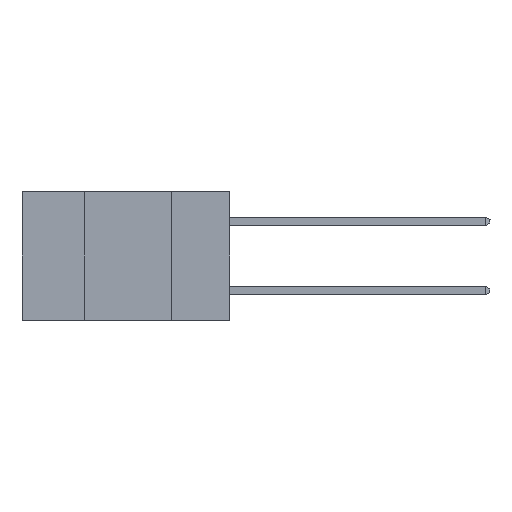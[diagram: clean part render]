
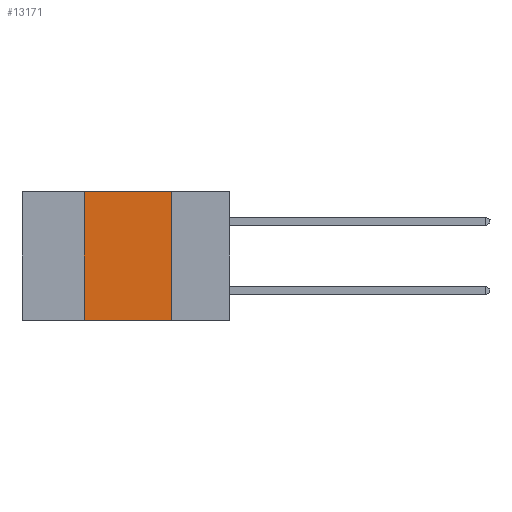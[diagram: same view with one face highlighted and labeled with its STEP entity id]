
A CAD part, left-side view. The second image highlights one B-rep face of the part: STEP entity #13171.
In plain terms, the highlighted planar face has unit normal (-1, 0, 0).
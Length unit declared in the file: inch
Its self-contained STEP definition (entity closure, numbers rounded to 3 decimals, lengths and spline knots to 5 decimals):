
#165 = CARTESIAN_POINT ( 'NONE',  ( 0., 0.42, -0.37 ) ) ;
#690 = VERTEX_POINT ( 'NONE', #16323 ) ;
#1790 = VECTOR ( 'NONE', #17800, 39.37008 ) ;
#2036 = CARTESIAN_POINT ( 'NONE',  ( 0., 0.17, -0.37 ) ) ;
#2674 = VECTOR ( 'NONE', #5970, 39.37008 ) ;
#3017 = EDGE_LOOP ( 'NONE', ( #17303, #17016, #16167, #13512 ) ) ;
#3249 = LINE ( 'NONE', #2036, #5496 ) ;
#3418 = CARTESIAN_POINT ( 'NONE',  ( 0., 0.42, 0. ) ) ;
#3550 = LINE ( 'NONE', #8054, #8302 ) ;
#4145 = EDGE_CURVE ( 'NONE', #10075, #17741, #3249, .T. ) ;
#4650 = CARTESIAN_POINT ( 'NONE',  ( 0., 0.17, -0.37 ) ) ;
#5496 = VECTOR ( 'NONE', #7744, 39.37008 ) ;
#5970 = DIRECTION ( 'NONE',  ( 0., 0., 1. ) ) ;
#6287 = CARTESIAN_POINT ( 'NONE',  ( 0., 0.17, 0. ) ) ;
#7280 = EDGE_CURVE ( 'NONE', #690, #11026, #10277, .T. ) ;
#7514 = FACE_OUTER_BOUND ( 'NONE', #3017, .T. ) ;
#7744 = DIRECTION ( 'NONE',  ( 0., 0., -1. ) ) ;
#7784 = EDGE_CURVE ( 'NONE', #11026, #10075, #7986, .T. ) ;
#7986 = LINE ( 'NONE', #16309, #1790 ) ;
#8054 = CARTESIAN_POINT ( 'NONE',  ( 0., 0.6, -0.37 ) ) ;
#8302 = VECTOR ( 'NONE', #13786, 39.37008 ) ;
#9024 = PLANE ( 'NONE',  #12723 ) ;
#10075 = VERTEX_POINT ( 'NONE', #6287 ) ;
#10277 = LINE ( 'NONE', #165, #2674 ) ;
#11026 = VERTEX_POINT ( 'NONE', #3418 ) ;
#11452 = DIRECTION ( 'NONE',  ( 1., 0., 0. ) ) ;
#12723 = AXIS2_PLACEMENT_3D ( 'NONE', #13331, #11452, #16220 ) ;
#13171 = ADVANCED_FACE ( 'NONE', ( #7514 ), #9024, .F. ) ;
#13331 = CARTESIAN_POINT ( 'NONE',  ( 0., 0.6, 0. ) ) ;
#13512 = ORIENTED_EDGE ( 'NONE', *, *, #18352, .T. ) ;
#13786 = DIRECTION ( 'NONE',  ( 0., -1., 0. ) ) ;
#16167 = ORIENTED_EDGE ( 'NONE', *, *, #7280, .F. ) ;
#16220 = DIRECTION ( 'NONE',  ( 0., 0., -1. ) ) ;
#16309 = CARTESIAN_POINT ( 'NONE',  ( 0., 0.6, 0. ) ) ;
#16323 = CARTESIAN_POINT ( 'NONE',  ( 0., 0.42, -0.37 ) ) ;
#17016 = ORIENTED_EDGE ( 'NONE', *, *, #7784, .F. ) ;
#17303 = ORIENTED_EDGE ( 'NONE', *, *, #4145, .F. ) ;
#17741 = VERTEX_POINT ( 'NONE', #4650 ) ;
#17800 = DIRECTION ( 'NONE',  ( 0., -1., 0. ) ) ;
#18352 = EDGE_CURVE ( 'NONE', #690, #17741, #3550, .T. ) ;
